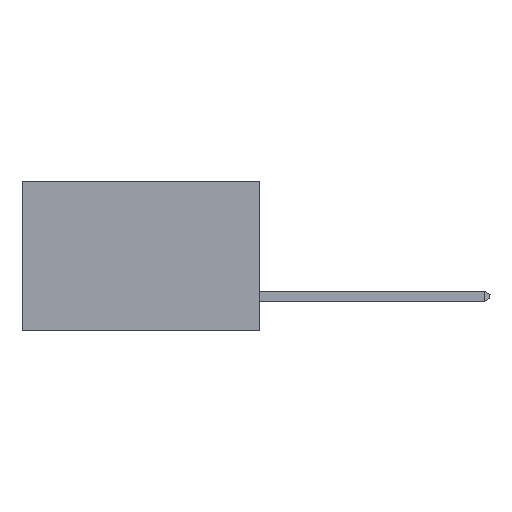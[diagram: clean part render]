
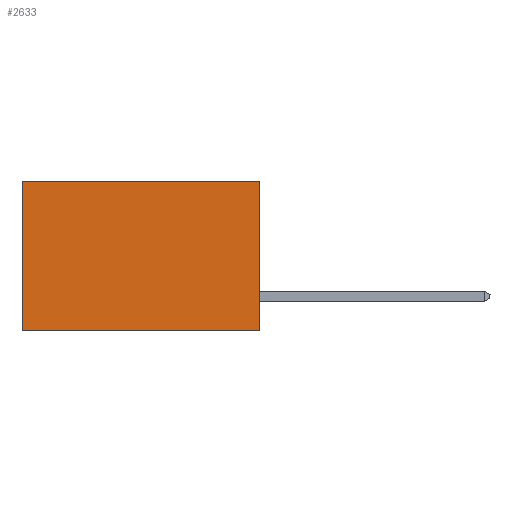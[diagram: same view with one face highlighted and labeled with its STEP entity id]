
A CAD part, left-side view. The second image highlights one B-rep face of the part: STEP entity #2633.
In plain terms, the highlighted planar face has unit normal (-1, 0, 0).
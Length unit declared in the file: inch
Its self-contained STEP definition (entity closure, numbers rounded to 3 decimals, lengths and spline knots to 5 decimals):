
#969 = CARTESIAN_POINT ( 'NONE',  ( 0.277, 0., -0.37 ) ) ;
#1429 = EDGE_CURVE ( 'NONE', #14090, #10731, #4498, .T. ) ;
#1457 = VECTOR ( 'NONE', #8498, 39.37008 ) ;
#1460 = EDGE_CURVE ( 'NONE', #9970, #13052, #4162, .T. ) ;
#1542 = VECTOR ( 'NONE', #8996, 39.37008 ) ;
#2633 = ADVANCED_FACE ( 'NONE', ( #6945 ), #9256, .F. ) ;
#3752 = ORIENTED_EDGE ( 'NONE', *, *, #1429, .T. ) ;
#3781 = EDGE_CURVE ( 'NONE', #13052, #10731, #7087, .T. ) ;
#3955 = ORIENTED_EDGE ( 'NONE', *, *, #3781, .F. ) ;
#4011 = ORIENTED_EDGE ( 'NONE', *, *, #1460, .F. ) ;
#4029 = ORIENTED_EDGE ( 'NONE', *, *, #4420, .T. ) ;
#4162 = LINE ( 'NONE', #8182, #1457 ) ;
#4420 = EDGE_CURVE ( 'NONE', #9970, #14090, #10436, .T. ) ;
#4498 = LINE ( 'NONE', #8411, #12727 ) ;
#6589 = CARTESIAN_POINT ( 'NONE',  ( 0.277, 0.59, -0.37 ) ) ;
#6945 = FACE_OUTER_BOUND ( 'NONE', #9499, .T. ) ;
#7087 = LINE ( 'NONE', #12634, #12339 ) ;
#8182 = CARTESIAN_POINT ( 'NONE',  ( 0.277, 0., -0.37 ) ) ;
#8298 = DIRECTION ( 'NONE',  ( 0., 0., -1. ) ) ;
#8411 = CARTESIAN_POINT ( 'NONE',  ( 0.277, 0.59, -0.37 ) ) ;
#8498 = DIRECTION ( 'NONE',  ( 0., 0., -1. ) ) ;
#8996 = DIRECTION ( 'NONE',  ( 0., 1., 0. ) ) ;
#8998 = DIRECTION ( 'NONE',  ( 0., 0., -1. ) ) ;
#9251 = CARTESIAN_POINT ( 'NONE',  ( 0.277, 0., 0. ) ) ;
#9256 = PLANE ( 'NONE',  #13067 ) ;
#9499 = EDGE_LOOP ( 'NONE', ( #3752, #3955, #4011, #4029 ) ) ;
#9970 = VERTEX_POINT ( 'NONE', #11577 ) ;
#10264 = DIRECTION ( 'NONE',  ( 0., 1., 0. ) ) ;
#10436 = LINE ( 'NONE', #9251, #1542 ) ;
#10731 = VERTEX_POINT ( 'NONE', #6589 ) ;
#10800 = DIRECTION ( 'NONE',  ( 1., 0., 0. ) ) ;
#11577 = CARTESIAN_POINT ( 'NONE',  ( 0.277, 0., 0. ) ) ;
#11653 = CARTESIAN_POINT ( 'NONE',  ( 0.277, 0., -0.37 ) ) ;
#12339 = VECTOR ( 'NONE', #10264, 39.37008 ) ;
#12634 = CARTESIAN_POINT ( 'NONE',  ( 0.277, 0., -0.37 ) ) ;
#12727 = VECTOR ( 'NONE', #8298, 39.37008 ) ;
#13052 = VERTEX_POINT ( 'NONE', #969 ) ;
#13067 = AXIS2_PLACEMENT_3D ( 'NONE', #11653, #10800, #8998 ) ;
#13723 = CARTESIAN_POINT ( 'NONE',  ( 0.277, 0.59, 0. ) ) ;
#14090 = VERTEX_POINT ( 'NONE', #13723 ) ;
